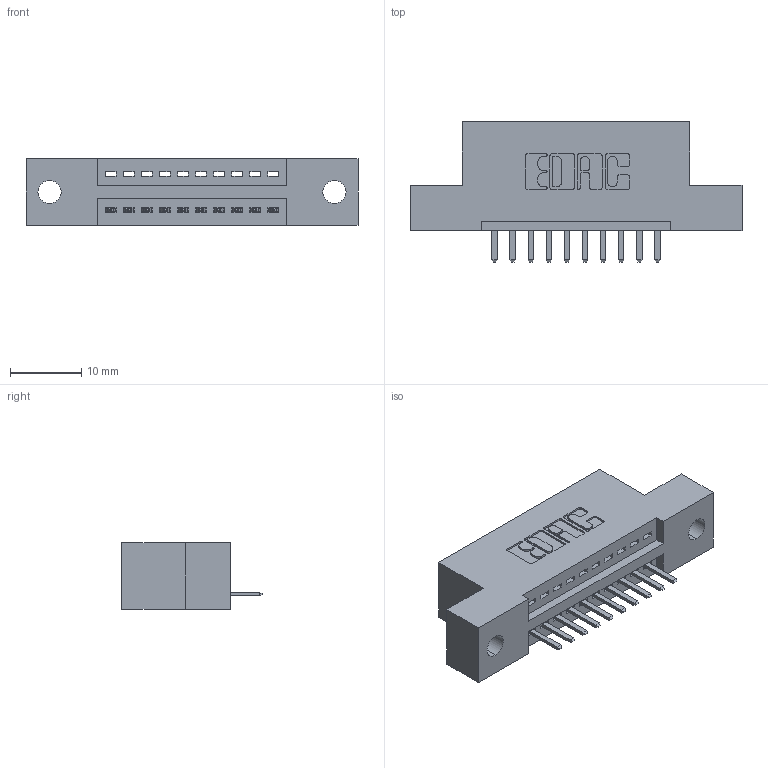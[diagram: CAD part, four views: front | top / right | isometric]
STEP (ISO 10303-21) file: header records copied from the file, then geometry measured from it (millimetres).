
FILE_DESCRIPTION (( 'STEP AP203' ), '1' );
FILE_NAME ('395-010-520-102.STEP', '2018-10-24T02:53:05', ( '' ), ( '' ), 'SwSTEP 2.0', 'SolidWorks 2016', '' );
FILE_SCHEMA (( 'CONFIG_CONTROL_DESIGN' ));
Length unit declared in the file: inch
Products named in the file (3): 395-010-520-102; 345 Part_Flush Mounting Lugs - 0.128 Dia; 345-292-001_345-293-120
Assembly tree (11 placements, depth 2):
  395-010-520-102
    345 Part_Flush Mounting Lugs - 0.128 Dia
    345-292-001_345-293-120  x10
Bounding box: 46.61 x 19.68 x 9.4 mm (x, y, z)
Volume: 4099.4 mm3; surface area: 4647.2 mm2
Topology: 11 solids, 11 shells, 746 faces, 2181 edges, 1426 vertices
Faces by surface type: plane 500, cylinder 246
Entity records: 11951 total; most frequent: CARTESIAN_POINT 2090, ORIENTED_EDGE 2022, DIRECTION 1859, EDGE_CURVE 1011, VECTOR 835, LINE 835, VERTEX_POINT 670, AXIS2_PLACEMENT_3D 512
